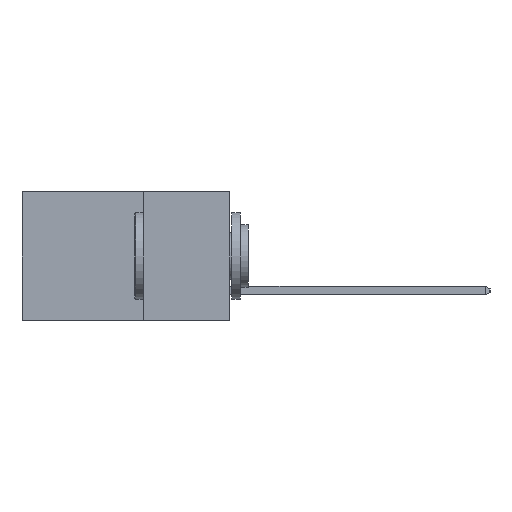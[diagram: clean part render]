
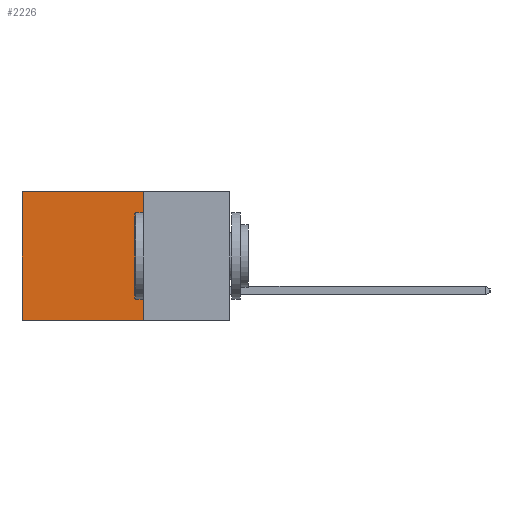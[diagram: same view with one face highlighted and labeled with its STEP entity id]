
A CAD part, left-side view. The second image highlights one B-rep face of the part: STEP entity #2226.
In plain terms, the highlighted planar face has unit normal (-1, 0, 0).
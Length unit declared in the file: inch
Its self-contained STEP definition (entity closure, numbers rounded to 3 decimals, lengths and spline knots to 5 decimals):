
#47 = AXIS2_PLACEMENT_3D ( 'NONE', #4672, #7737, #8940 ) ;
#299 = VERTEX_POINT ( 'NONE', #3000 ) ;
#337 = DIRECTION ( 'NONE',  ( 0., 0., -1. ) ) ;
#366 = EDGE_CURVE ( 'NONE', #5340, #299, #7072, .T. ) ;
#1569 = LINE ( 'NONE', #10070, #7678 ) ;
#1695 = CARTESIAN_POINT ( 'NONE',  ( 0.2615, 0.25, 0. ) ) ;
#1713 = DIRECTION ( 'NONE',  ( 0., 1., 0. ) ) ;
#1900 = FACE_OUTER_BOUND ( 'NONE', #5267, .T. ) ;
#2012 = EDGE_CURVE ( 'NONE', #5527, #3508, #10143, .T. ) ;
#2226 = ADVANCED_FACE ( 'NONE', ( #1900 ), #7757, .F. ) ;
#3000 = CARTESIAN_POINT ( 'NONE',  ( 0.2615, 0.6, -0.37 ) ) ;
#3006 = CARTESIAN_POINT ( 'NONE',  ( 0.2615, 0.6, -0.37 ) ) ;
#3348 = ORIENTED_EDGE ( 'NONE', *, *, #366, .T. ) ;
#3508 = VERTEX_POINT ( 'NONE', #4366 ) ;
#3564 = LINE ( 'NONE', #1695, #5971 ) ;
#3926 = VECTOR ( 'NONE', #7400, 39.37008 ) ;
#4116 = CARTESIAN_POINT ( 'NONE',  ( 0.2615, 0.25, 0. ) ) ;
#4366 = CARTESIAN_POINT ( 'NONE',  ( 0.2615, 0.25, -0.37 ) ) ;
#4672 = CARTESIAN_POINT ( 'NONE',  ( 0.2615, 0.25, -0.37 ) ) ;
#5028 = VECTOR ( 'NONE', #337, 39.37008 ) ;
#5267 = EDGE_LOOP ( 'NONE', ( #3348, #5523, #7581, #9613 ) ) ;
#5340 = VERTEX_POINT ( 'NONE', #5437 ) ;
#5437 = CARTESIAN_POINT ( 'NONE',  ( 0.2615, 0.6, 0. ) ) ;
#5523 = ORIENTED_EDGE ( 'NONE', *, *, #5992, .F. ) ;
#5527 = VERTEX_POINT ( 'NONE', #4116 ) ;
#5796 = EDGE_CURVE ( 'NONE', #5527, #5340, #3564, .T. ) ;
#5971 = VECTOR ( 'NONE', #1713, 39.37008 ) ;
#5992 = EDGE_CURVE ( 'NONE', #3508, #299, #1569, .T. ) ;
#7072 = LINE ( 'NONE', #3006, #5028 ) ;
#7400 = DIRECTION ( 'NONE',  ( 0., 0., -1. ) ) ;
#7581 = ORIENTED_EDGE ( 'NONE', *, *, #2012, .F. ) ;
#7678 = VECTOR ( 'NONE', #9952, 39.37008 ) ;
#7737 = DIRECTION ( 'NONE',  ( 1., 0., 0. ) ) ;
#7757 = PLANE ( 'NONE',  #47 ) ;
#8940 = DIRECTION ( 'NONE',  ( 0., 0., -1. ) ) ;
#9613 = ORIENTED_EDGE ( 'NONE', *, *, #5796, .T. ) ;
#9665 = CARTESIAN_POINT ( 'NONE',  ( 0.2615, 0.25, -0.37 ) ) ;
#9952 = DIRECTION ( 'NONE',  ( 0., 1., 0. ) ) ;
#10070 = CARTESIAN_POINT ( 'NONE',  ( 0.2615, 0.25, -0.37 ) ) ;
#10143 = LINE ( 'NONE', #9665, #3926 ) ;
